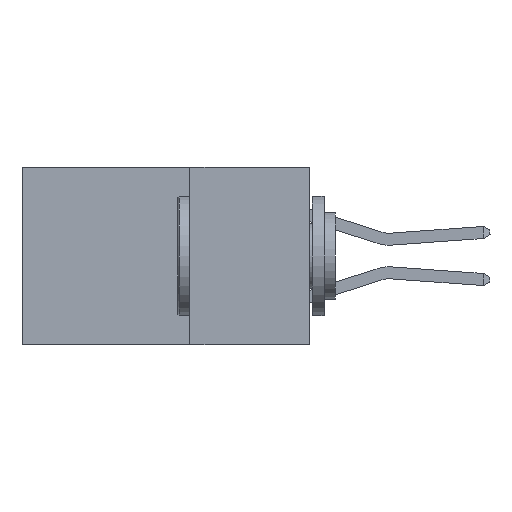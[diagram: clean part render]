
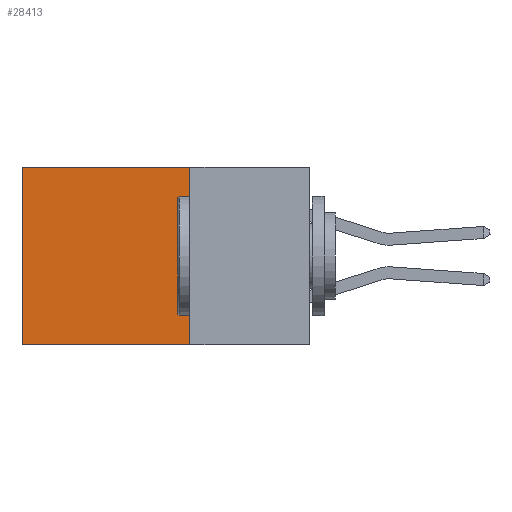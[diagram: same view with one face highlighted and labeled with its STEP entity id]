
A CAD part, left-side view. The second image highlights one B-rep face of the part: STEP entity #28413.
In plain terms, the highlighted planar face has unit normal (-1, 0, 0).
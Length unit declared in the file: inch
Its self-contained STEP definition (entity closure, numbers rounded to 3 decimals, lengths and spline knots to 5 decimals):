
#160 = EDGE_LOOP ( 'NONE', ( #18397, #6070, #1008, #3991 ) ) ;
#184 = CARTESIAN_POINT ( 'NONE',  ( 0.298, 0.25, -0.37 ) ) ;
#376 = CARTESIAN_POINT ( 'NONE',  ( 0.298, 0.25, 0. ) ) ;
#1008 = ORIENTED_EDGE ( 'NONE', *, *, #25387, .F. ) ;
#1270 = PLANE ( 'NONE',  #28862 ) ;
#2012 = CARTESIAN_POINT ( 'NONE',  ( 0.298, 0.6, -0.37 ) ) ;
#3713 = DIRECTION ( 'NONE',  ( 1., 0., 0. ) ) ;
#3991 = ORIENTED_EDGE ( 'NONE', *, *, #15129, .T. ) ;
#4856 = CARTESIAN_POINT ( 'NONE',  ( 0.298, 0.25, 0. ) ) ;
#5451 = CARTESIAN_POINT ( 'NONE',  ( 0.298, 0.6, 0. ) ) ;
#6037 = CARTESIAN_POINT ( 'NONE',  ( 0.298, 0.25, 0. ) ) ;
#6070 = ORIENTED_EDGE ( 'NONE', *, *, #13530, .F. ) ;
#6608 = CARTESIAN_POINT ( 'NONE',  ( 0.298, 0.25, 0. ) ) ;
#7508 = DIRECTION ( 'NONE',  ( 0., 0., -1. ) ) ;
#7603 = VECTOR ( 'NONE', #14161, 39.37008 ) ;
#7665 = DIRECTION ( 'NONE',  ( 0., 0., -1. ) ) ;
#8345 = LINE ( 'NONE', #4856, #7603 ) ;
#10097 = VERTEX_POINT ( 'NONE', #184 ) ;
#10310 = VECTOR ( 'NONE', #25806, 39.37008 ) ;
#10782 = VERTEX_POINT ( 'NONE', #5451 ) ;
#11418 = EDGE_CURVE ( 'NONE', #10782, #17720, #21713, .T. ) ;
#12098 = VERTEX_POINT ( 'NONE', #6608 ) ;
#13530 = EDGE_CURVE ( 'NONE', #10097, #17720, #28600, .T. ) ;
#14161 = DIRECTION ( 'NONE',  ( 0., 1., 0. ) ) ;
#14320 = CARTESIAN_POINT ( 'NONE',  ( 0.298, 0.6, 0. ) ) ;
#15129 = EDGE_CURVE ( 'NONE', #12098, #10782, #8345, .T. ) ;
#15555 = VECTOR ( 'NONE', #7508, 39.37008 ) ;
#16600 = CARTESIAN_POINT ( 'NONE',  ( 0.298, 0.25, -0.37 ) ) ;
#17720 = VERTEX_POINT ( 'NONE', #2012 ) ;
#18397 = ORIENTED_EDGE ( 'NONE', *, *, #11418, .T. ) ;
#20005 = FACE_OUTER_BOUND ( 'NONE', #160, .T. ) ;
#20092 = DIRECTION ( 'NONE',  ( 0., 0., -1. ) ) ;
#20507 = LINE ( 'NONE', #376, #21236 ) ;
#21236 = VECTOR ( 'NONE', #7665, 39.37008 ) ;
#21713 = LINE ( 'NONE', #14320, #15555 ) ;
#25387 = EDGE_CURVE ( 'NONE', #12098, #10097, #20507, .T. ) ;
#25806 = DIRECTION ( 'NONE',  ( 0., 1., 0. ) ) ;
#28413 = ADVANCED_FACE ( 'NONE', ( #20005 ), #1270, .F. ) ;
#28600 = LINE ( 'NONE', #16600, #10310 ) ;
#28862 = AXIS2_PLACEMENT_3D ( 'NONE', #6037, #3713, #20092 ) ;
